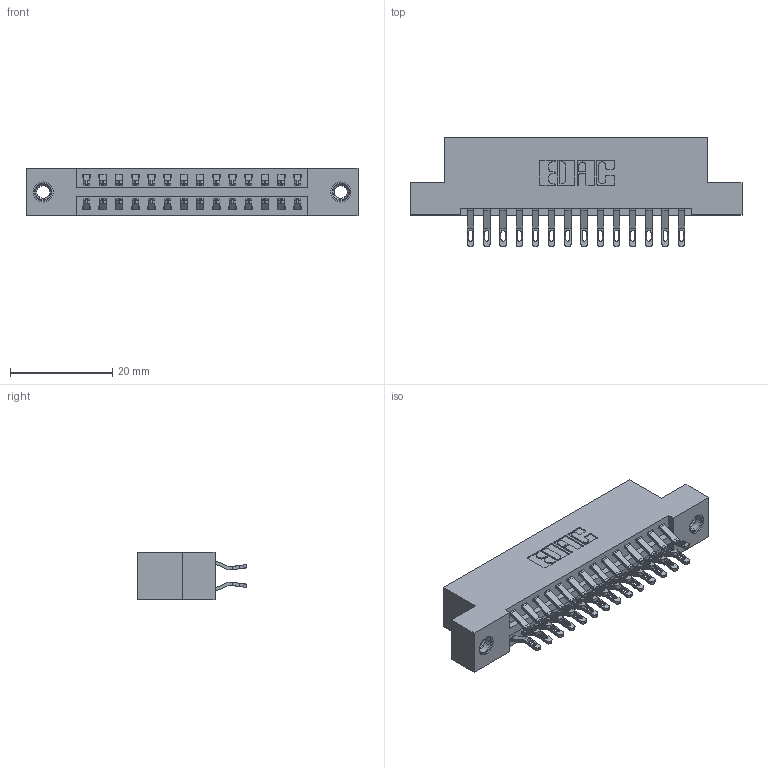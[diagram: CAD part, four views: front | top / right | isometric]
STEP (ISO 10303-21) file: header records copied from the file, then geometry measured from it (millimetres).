
FILE_DESCRIPTION (( 'STEP AP203' ), '1' );
FILE_NAME ('396-028-555-207.STEP', '2019-10-30T05:23:18', ( '' ), ( '' ), 'SwSTEP 2.0', 'SolidWorks 2016', '' );
FILE_SCHEMA (( 'CONFIG_CONTROL_DESIGN' ));
Length unit declared in the file: inch
Products named in the file (4): 345-250-001_345-250-005-103; 345-292-001_555 Tail; 396-028-555-207; 346 Part_Flush Mounting Lugs - 0.156 Dia-TI
Assembly tree (31 placements, depth 2):
  396-028-555-207
    346 Part_Flush Mounting Lugs - 0.156 Dia-TI
    345-292-001_555 Tail  x28
    345-250-001_345-250-005-103  x2
Bounding box: 65.02 x 21.46 x 9.4 mm (x, y, z)
Volume: 6190.9 mm3; surface area: 8392.9 mm2
Topology: 31 solids, 31 shells, 1806 faces, 5589 edges, 3718 vertices
Faces by surface type: plane 1032, cylinder 758, cone 12, torus 4
Entity records: 14418 total; most frequent: CARTESIAN_POINT 2433, ORIENTED_EDGE 2330, DIRECTION 2191, EDGE_CURVE 1165, LINE 937, VECTOR 937, VERTEX_POINT 772, AXIS2_PLACEMENT_3D 627
